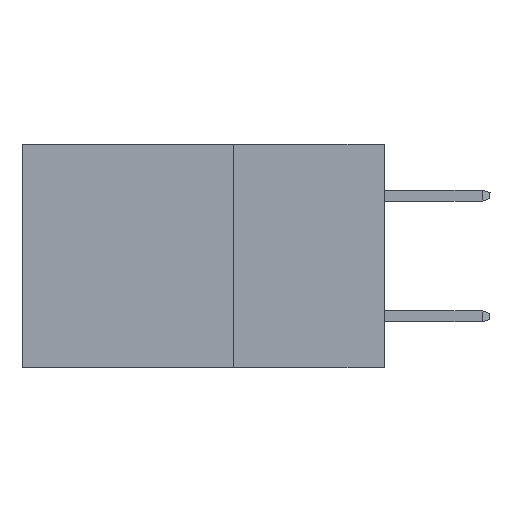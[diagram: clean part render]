
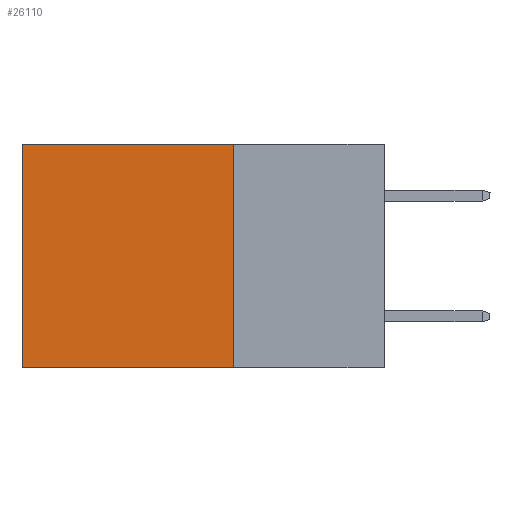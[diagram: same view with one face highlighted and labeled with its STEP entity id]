
A CAD part, left-side view. The second image highlights one B-rep face of the part: STEP entity #26110.
In plain terms, the highlighted planar face has unit normal (-1, 0, 0).
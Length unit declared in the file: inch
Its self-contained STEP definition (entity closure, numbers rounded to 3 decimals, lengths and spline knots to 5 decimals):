
#1140 = DIRECTION ( 'NONE',  ( 0., 1., 0. ) ) ;
#1804 = DIRECTION ( 'NONE',  ( 0., 1., 0. ) ) ;
#2449 = VERTEX_POINT ( 'NONE', #26166 ) ;
#4498 = CARTESIAN_POINT ( 'NONE',  ( 0.298, 0.25, 0. ) ) ;
#4593 = VECTOR ( 'NONE', #1804, 39.37008 ) ;
#5784 = ORIENTED_EDGE ( 'NONE', *, *, #7635, .F. ) ;
#6100 = CARTESIAN_POINT ( 'NONE',  ( 0.298, 0.25, -0.37 ) ) ;
#6314 = DIRECTION ( 'NONE',  ( 0., 0., -1. ) ) ;
#7449 = EDGE_LOOP ( 'NONE', ( #23852, #5784, #17961, #16321 ) ) ;
#7635 = EDGE_CURVE ( 'NONE', #16045, #20197, #8051, .T. ) ;
#7927 = VECTOR ( 'NONE', #12643, 39.37008 ) ;
#8051 = LINE ( 'NONE', #6100, #4593 ) ;
#8118 = VERTEX_POINT ( 'NONE', #9997 ) ;
#8818 = CARTESIAN_POINT ( 'NONE',  ( 0.298, 0.6, -0.37 ) ) ;
#9997 = CARTESIAN_POINT ( 'NONE',  ( 0.298, 0.25, 0. ) ) ;
#10541 = DIRECTION ( 'NONE',  ( 0., 0., -1. ) ) ;
#12643 = DIRECTION ( 'NONE',  ( 0., 0., -1. ) ) ;
#13161 = VECTOR ( 'NONE', #6314, 39.37008 ) ;
#13505 = LINE ( 'NONE', #20392, #13161 ) ;
#13530 = EDGE_CURVE ( 'NONE', #2449, #20197, #13505, .T. ) ;
#14633 = LINE ( 'NONE', #20787, #7927 ) ;
#14724 = LINE ( 'NONE', #23581, #23549 ) ;
#16045 = VERTEX_POINT ( 'NONE', #21005 ) ;
#16321 = ORIENTED_EDGE ( 'NONE', *, *, #23598, .T. ) ;
#16527 = DIRECTION ( 'NONE',  ( 1., 0., 0. ) ) ;
#17558 = AXIS2_PLACEMENT_3D ( 'NONE', #4498, #16527, #10541 ) ;
#17961 = ORIENTED_EDGE ( 'NONE', *, *, #19686, .F. ) ;
#18820 = PLANE ( 'NONE',  #17558 ) ;
#19686 = EDGE_CURVE ( 'NONE', #8118, #16045, #14633, .T. ) ;
#20197 = VERTEX_POINT ( 'NONE', #8818 ) ;
#20392 = CARTESIAN_POINT ( 'NONE',  ( 0.298, 0.6, 0. ) ) ;
#20787 = CARTESIAN_POINT ( 'NONE',  ( 0.298, 0.25, 0. ) ) ;
#21005 = CARTESIAN_POINT ( 'NONE',  ( 0.298, 0.25, -0.37 ) ) ;
#22759 = FACE_OUTER_BOUND ( 'NONE', #7449, .T. ) ;
#23549 = VECTOR ( 'NONE', #1140, 39.37008 ) ;
#23581 = CARTESIAN_POINT ( 'NONE',  ( 0.298, 0.25, 0. ) ) ;
#23598 = EDGE_CURVE ( 'NONE', #8118, #2449, #14724, .T. ) ;
#23852 = ORIENTED_EDGE ( 'NONE', *, *, #13530, .T. ) ;
#26110 = ADVANCED_FACE ( 'NONE', ( #22759 ), #18820, .F. ) ;
#26166 = CARTESIAN_POINT ( 'NONE',  ( 0.298, 0.6, 0. ) ) ;
